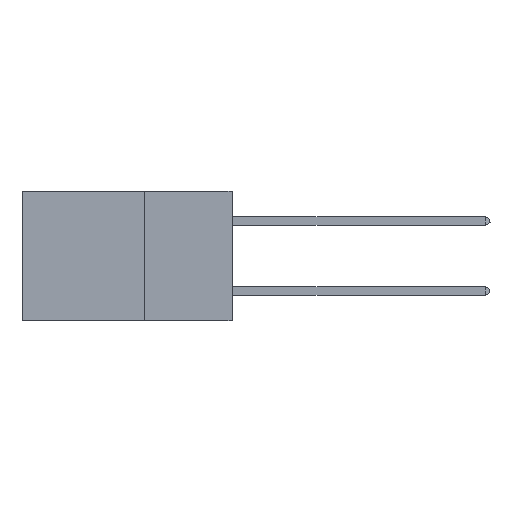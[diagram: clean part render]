
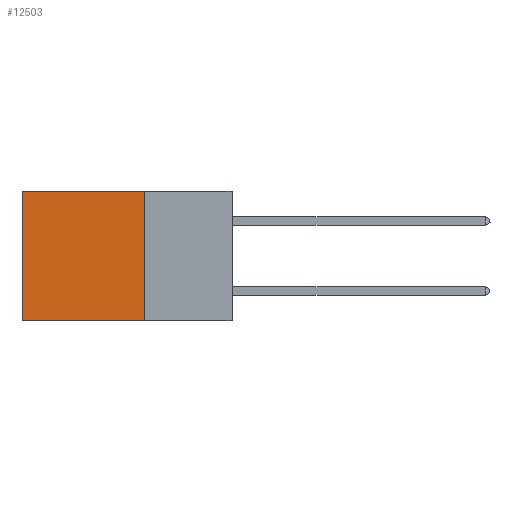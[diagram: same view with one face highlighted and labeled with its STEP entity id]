
A CAD part, left-side view. The second image highlights one B-rep face of the part: STEP entity #12503.
In plain terms, the highlighted planar face has unit normal (-1, 0, 0).
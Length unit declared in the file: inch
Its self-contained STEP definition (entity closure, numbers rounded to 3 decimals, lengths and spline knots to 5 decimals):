
#72 = LINE ( 'NONE', #5435, #19533 ) ;
#619 = CARTESIAN_POINT ( 'NONE',  ( 0.2875, 0.25, -0.37 ) ) ;
#1858 = EDGE_CURVE ( 'NONE', #20558, #11214, #17392, .T. ) ;
#1922 = DIRECTION ( 'NONE',  ( 0., 0., -1. ) ) ;
#2001 = VERTEX_POINT ( 'NONE', #22161 ) ;
#2816 = EDGE_CURVE ( 'NONE', #11214, #13773, #72, .T. ) ;
#2916 = PLANE ( 'NONE',  #8312 ) ;
#3118 = EDGE_CURVE ( 'NONE', #20558, #2001, #5177, .T. ) ;
#3223 = CARTESIAN_POINT ( 'NONE',  ( 0.2875, 0.25, 0. ) ) ;
#3333 = CARTESIAN_POINT ( 'NONE',  ( 0.2875, 0.25, 0. ) ) ;
#4133 = EDGE_LOOP ( 'NONE', ( #11149, #5573, #8880, #7718 ) ) ;
#5177 = LINE ( 'NONE', #12597, #17670 ) ;
#5185 = CARTESIAN_POINT ( 'NONE',  ( 0.2875, 0.25, 0. ) ) ;
#5435 = CARTESIAN_POINT ( 'NONE',  ( 0.2875, 0.6, 0. ) ) ;
#5573 = ORIENTED_EDGE ( 'NONE', *, *, #8807, .F. ) ;
#7718 = ORIENTED_EDGE ( 'NONE', *, *, #1858, .T. ) ;
#8312 = AXIS2_PLACEMENT_3D ( 'NONE', #5185, #12736, #21759 ) ;
#8807 = EDGE_CURVE ( 'NONE', #2001, #13773, #20524, .T. ) ;
#8880 = ORIENTED_EDGE ( 'NONE', *, *, #3118, .F. ) ;
#10843 = CARTESIAN_POINT ( 'NONE',  ( 0.2875, 0.6, 0. ) ) ;
#11149 = ORIENTED_EDGE ( 'NONE', *, *, #2816, .T. ) ;
#11214 = VERTEX_POINT ( 'NONE', #10843 ) ;
#11662 = DIRECTION ( 'NONE',  ( 0., 1., 0. ) ) ;
#12503 = ADVANCED_FACE ( 'NONE', ( #20922 ), #2916, .F. ) ;
#12510 = DIRECTION ( 'NONE',  ( 0., 0., -1. ) ) ;
#12597 = CARTESIAN_POINT ( 'NONE',  ( 0.2875, 0.25, 0. ) ) ;
#12736 = DIRECTION ( 'NONE',  ( 1., 0., 0. ) ) ;
#12755 = VECTOR ( 'NONE', #11662, 39.37008 ) ;
#13773 = VERTEX_POINT ( 'NONE', #14470 ) ;
#14470 = CARTESIAN_POINT ( 'NONE',  ( 0.2875, 0.6, -0.37 ) ) ;
#17392 = LINE ( 'NONE', #3333, #19937 ) ;
#17503 = DIRECTION ( 'NONE',  ( 0., 1., 0. ) ) ;
#17670 = VECTOR ( 'NONE', #1922, 39.37008 ) ;
#19533 = VECTOR ( 'NONE', #12510, 39.37008 ) ;
#19937 = VECTOR ( 'NONE', #17503, 39.37008 ) ;
#20524 = LINE ( 'NONE', #619, #12755 ) ;
#20558 = VERTEX_POINT ( 'NONE', #3223 ) ;
#20922 = FACE_OUTER_BOUND ( 'NONE', #4133, .T. ) ;
#21759 = DIRECTION ( 'NONE',  ( 0., 0., -1. ) ) ;
#22161 = CARTESIAN_POINT ( 'NONE',  ( 0.2875, 0.25, -0.37 ) ) ;
